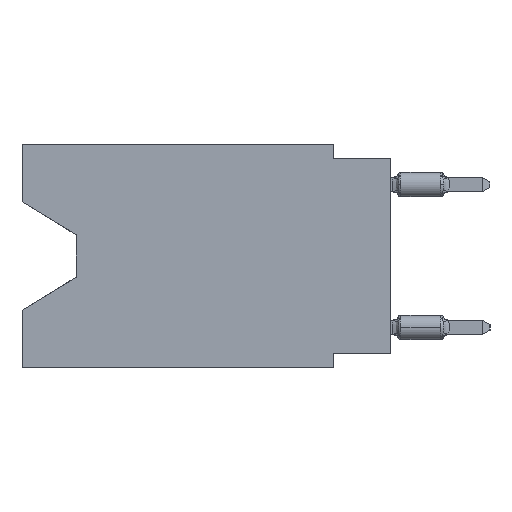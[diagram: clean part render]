
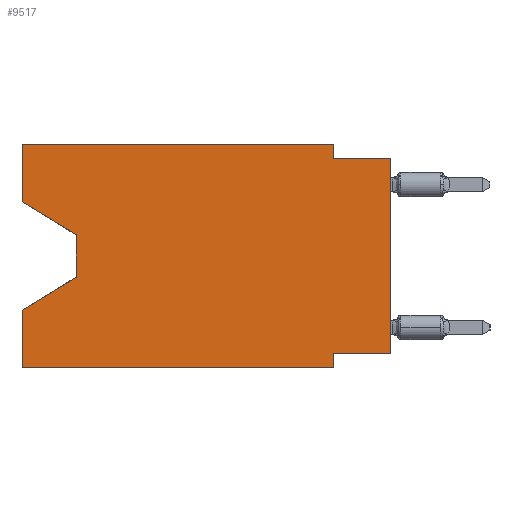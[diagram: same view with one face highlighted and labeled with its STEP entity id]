
A CAD part, left-side view. The second image highlights one B-rep face of the part: STEP entity #9517.
In plain terms, the highlighted planar face has unit normal (-1, 0, 0).
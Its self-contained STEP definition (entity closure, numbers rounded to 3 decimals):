
#134 = PLANE ( 'NONE',  #2737 ) ;
#436 = CARTESIAN_POINT ( 'NONE',  ( 0., 16.383, 0. ) ) ;
#603 = VERTEX_POINT ( 'NONE', #20714 ) ;
#1493 = VERTEX_POINT ( 'NONE', #23482 ) ;
#2440 = CARTESIAN_POINT ( 'NONE',  ( 0., 2.54, 0. ) ) ;
#2649 = DIRECTION ( 'NONE',  ( 0., 1., 0. ) ) ;
#2737 = AXIS2_PLACEMENT_3D ( 'NONE', #436, #18822, #6939 ) ;
#2972 = VECTOR ( 'NONE', #20701, 1000. ) ;
#3596 = ORIENTED_EDGE ( 'NONE', *, *, #16831, .F. ) ;
#3686 = LINE ( 'NONE', #9221, #26660 ) ;
#3749 = VERTEX_POINT ( 'NONE', #8637 ) ;
#4041 = VECTOR ( 'NONE', #25854, 1000. ) ;
#4266 = LINE ( 'NONE', #11369, #7375 ) ;
#4436 = CARTESIAN_POINT ( 'NONE',  ( 0., 0., -0.635 ) ) ;
#4716 = CARTESIAN_POINT ( 'NONE',  ( 0., 2.54, 0. ) ) ;
#4970 = VECTOR ( 'NONE', #6391, 1000. ) ;
#5071 = EDGE_CURVE ( 'NONE', #19543, #14220, #28196, .T. ) ;
#5115 = EDGE_CURVE ( 'NONE', #14220, #20157, #26379, .T. ) ;
#6391 = DIRECTION ( 'NONE',  ( 0., 0., 1. ) ) ;
#6492 = ORIENTED_EDGE ( 'NONE', *, *, #11900, .T. ) ;
#6539 = LINE ( 'NONE', #17683, #16151 ) ;
#6826 = LINE ( 'NONE', #25234, #14605 ) ;
#6939 = DIRECTION ( 'NONE',  ( 0., 0., -1. ) ) ;
#7319 = CARTESIAN_POINT ( 'NONE',  ( 0., 0., -9.271 ) ) ;
#7375 = VECTOR ( 'NONE', #22822, 1000. ) ;
#7736 = CARTESIAN_POINT ( 'NONE',  ( 0., 0., -9.271 ) ) ;
#8510 = LINE ( 'NONE', #24189, #28902 ) ;
#8637 = CARTESIAN_POINT ( 'NONE',  ( 0., 2.54, -0.635 ) ) ;
#9221 = CARTESIAN_POINT ( 'NONE',  ( 0., 13.97, -5.893 ) ) ;
#9236 = CARTESIAN_POINT ( 'NONE',  ( 0., 16.383, -2.546 ) ) ;
#9517 = ADVANCED_FACE ( 'NONE', ( #21091 ), #134, .F. ) ;
#9747 = VECTOR ( 'NONE', #14900, 1000. ) ;
#10307 = VERTEX_POINT ( 'NONE', #11527 ) ;
#10492 = EDGE_CURVE ( 'NONE', #20602, #1493, #26446, .T. ) ;
#11369 = CARTESIAN_POINT ( 'NONE',  ( 0., 16.383, -9.906 ) ) ;
#11429 = ORIENTED_EDGE ( 'NONE', *, *, #25866, .F. ) ;
#11504 = DIRECTION ( 'NONE',  ( 0., 0., -1. ) ) ;
#11527 = CARTESIAN_POINT ( 'NONE',  ( 0., 16.383, 0. ) ) ;
#11532 = CARTESIAN_POINT ( 'NONE',  ( 0., 2.54, -9.271 ) ) ;
#11900 = EDGE_CURVE ( 'NONE', #20157, #1493, #3686, .T. ) ;
#12053 = CARTESIAN_POINT ( 'NONE',  ( 0., 16.383, -2.546 ) ) ;
#12105 = LINE ( 'NONE', #2440, #27608 ) ;
#12126 = ORIENTED_EDGE ( 'NONE', *, *, #5071, .T. ) ;
#12193 = ORIENTED_EDGE ( 'NONE', *, *, #28289, .F. ) ;
#12381 = CARTESIAN_POINT ( 'NONE',  ( 0., 16.383, -9.906 ) ) ;
#13164 = VERTEX_POINT ( 'NONE', #7736 ) ;
#13411 = ORIENTED_EDGE ( 'NONE', *, *, #21834, .F. ) ;
#14164 = DIRECTION ( 'NONE',  ( 0., -0.855, -0.519 ) ) ;
#14220 = VERTEX_POINT ( 'NONE', #24524 ) ;
#14605 = VECTOR ( 'NONE', #29732, 1000. ) ;
#14660 = CARTESIAN_POINT ( 'NONE',  ( 0., 2.54, -9.906 ) ) ;
#14900 = DIRECTION ( 'NONE',  ( 0., 0., -1. ) ) ;
#15414 = LINE ( 'NONE', #24626, #4970 ) ;
#15817 = ORIENTED_EDGE ( 'NONE', *, *, #18112, .T. ) ;
#16151 = VECTOR ( 'NONE', #29149, 1000. ) ;
#16491 = LINE ( 'NONE', #4436, #2972 ) ;
#16655 = CARTESIAN_POINT ( 'NONE',  ( 0., 16.383, 0. ) ) ;
#16831 = EDGE_CURVE ( 'NONE', #10307, #29651, #6539, .T. ) ;
#17680 = DIRECTION ( 'NONE',  ( 0., 0., -1. ) ) ;
#17683 = CARTESIAN_POINT ( 'NONE',  ( 0., 16.383, 0. ) ) ;
#18112 = EDGE_CURVE ( 'NONE', #20602, #27656, #4266, .T. ) ;
#18222 = EDGE_CURVE ( 'NONE', #13164, #603, #6826, .T. ) ;
#18822 = DIRECTION ( 'NONE',  ( 1., 0., 0. ) ) ;
#19414 = ORIENTED_EDGE ( 'NONE', *, *, #21623, .F. ) ;
#19543 = VERTEX_POINT ( 'NONE', #9236 ) ;
#20157 = VERTEX_POINT ( 'NONE', #21581 ) ;
#20602 = VERTEX_POINT ( 'NONE', #12381 ) ;
#20701 = DIRECTION ( 'NONE',  ( 0., -1., 0. ) ) ;
#20714 = CARTESIAN_POINT ( 'NONE',  ( 0., 0., -0.635 ) ) ;
#21064 = EDGE_LOOP ( 'NONE', ( #12126, #22323, #6492, #25579, #15817, #12193, #29810, #24331, #11429, #13411, #3596, #19414 ) ) ;
#21091 = FACE_OUTER_BOUND ( 'NONE', #21064, .T. ) ;
#21450 = EDGE_CURVE ( 'NONE', #13164, #29229, #28135, .T. ) ;
#21581 = CARTESIAN_POINT ( 'NONE',  ( 0., 13.97, -5.893 ) ) ;
#21623 = EDGE_CURVE ( 'NONE', #19543, #10307, #15414, .T. ) ;
#21834 = EDGE_CURVE ( 'NONE', #29651, #3749, #12105, .T. ) ;
#22323 = ORIENTED_EDGE ( 'NONE', *, *, #5115, .T. ) ;
#22822 = DIRECTION ( 'NONE',  ( 0., -1., 0. ) ) ;
#23482 = CARTESIAN_POINT ( 'NONE',  ( 0., 16.383, -7.36 ) ) ;
#24189 = CARTESIAN_POINT ( 'NONE',  ( 0., 2.54, -9.906 ) ) ;
#24331 = ORIENTED_EDGE ( 'NONE', *, *, #18222, .T. ) ;
#24524 = CARTESIAN_POINT ( 'NONE',  ( 0., 13.97, -4.013 ) ) ;
#24626 = CARTESIAN_POINT ( 'NONE',  ( 0., 16.383, 0. ) ) ;
#25234 = CARTESIAN_POINT ( 'NONE',  ( 0., 0., 0. ) ) ;
#25579 = ORIENTED_EDGE ( 'NONE', *, *, #10492, .F. ) ;
#25854 = DIRECTION ( 'NONE',  ( 0., 0., 1. ) ) ;
#25866 = EDGE_CURVE ( 'NONE', #3749, #603, #16491, .T. ) ;
#26379 = LINE ( 'NONE', #28630, #9747 ) ;
#26446 = LINE ( 'NONE', #16655, #4041 ) ;
#26660 = VECTOR ( 'NONE', #27919, 1000. ) ;
#27122 = VECTOR ( 'NONE', #2649, 1000. ) ;
#27515 = VECTOR ( 'NONE', #14164, 1000. ) ;
#27608 = VECTOR ( 'NONE', #11504, 1000. ) ;
#27656 = VERTEX_POINT ( 'NONE', #14660 ) ;
#27919 = DIRECTION ( 'NONE',  ( 0., 0.855, -0.519 ) ) ;
#28135 = LINE ( 'NONE', #7319, #27122 ) ;
#28196 = LINE ( 'NONE', #12053, #27515 ) ;
#28289 = EDGE_CURVE ( 'NONE', #29229, #27656, #8510, .T. ) ;
#28630 = CARTESIAN_POINT ( 'NONE',  ( 0., 13.97, -4.013 ) ) ;
#28902 = VECTOR ( 'NONE', #17680, 1000. ) ;
#29149 = DIRECTION ( 'NONE',  ( 0., -1., 0. ) ) ;
#29229 = VERTEX_POINT ( 'NONE', #11532 ) ;
#29651 = VERTEX_POINT ( 'NONE', #4716 ) ;
#29732 = DIRECTION ( 'NONE',  ( 0., 0., 1. ) ) ;
#29810 = ORIENTED_EDGE ( 'NONE', *, *, #21450, .F. ) ;
